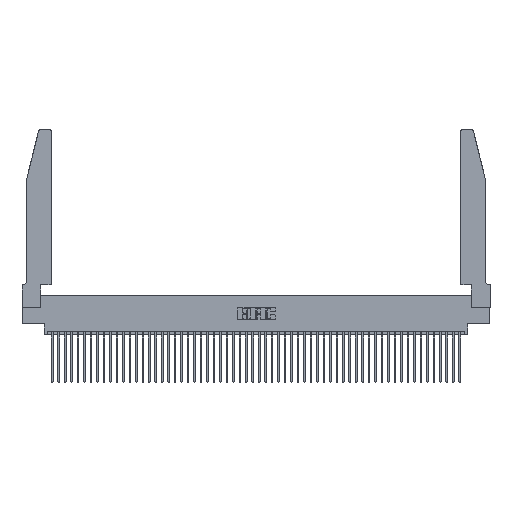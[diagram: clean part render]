
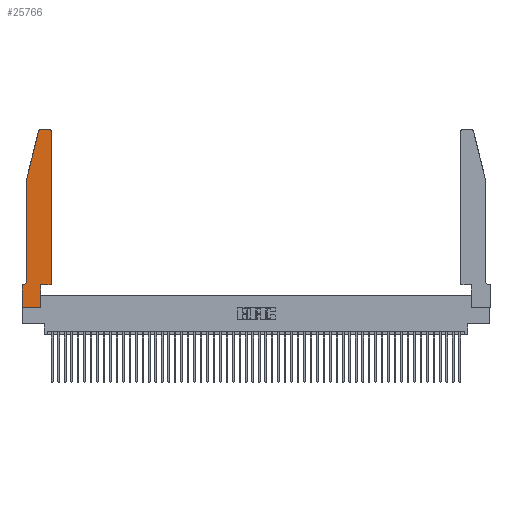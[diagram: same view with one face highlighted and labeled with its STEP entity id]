
A CAD part, top view. The second image highlights one B-rep face of the part: STEP entity #25766.
In plain terms, the highlighted planar face has unit normal (0, 0, 1).
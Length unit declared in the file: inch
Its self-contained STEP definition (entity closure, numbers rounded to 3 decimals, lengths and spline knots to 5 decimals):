
#330 = DIRECTION ( 'NONE',  ( 0., 0., 1. ) ) ;
#404 = VECTOR ( 'NONE', #18850, 39.37008 ) ;
#781 = CARTESIAN_POINT ( 'NONE',  ( 0.284, 2.75, 0.37 ) ) ;
#1384 = CIRCLE ( 'NONE', #18225, 0.03 ) ;
#3979 = EDGE_CURVE ( 'NONE', #7388, #43879, #4180, .T. ) ;
#4016 = VERTEX_POINT ( 'NONE', #40370 ) ;
#4180 = LINE ( 'NONE', #6668, #404 ) ;
#4726 = VECTOR ( 'NONE', #18629, 39.37008 ) ;
#5126 = DIRECTION ( 'NONE',  ( 1., 0., 0. ) ) ;
#5269 = EDGE_CURVE ( 'NONE', #43879, #4016, #16724, .T. ) ;
#5546 = CARTESIAN_POINT ( 'NONE',  ( 0., 0., 0.37 ) ) ;
#5637 = EDGE_CURVE ( 'NONE', #10008, #19108, #41903, .T. ) ;
#6426 = CARTESIAN_POINT ( 'NONE',  ( 0.0755, 2., 0.37 ) ) ;
#6668 = CARTESIAN_POINT ( 'NONE',  ( 0., 0., 0.37 ) ) ;
#7388 = VERTEX_POINT ( 'NONE', #5546 ) ;
#8539 = CARTESIAN_POINT ( 'NONE',  ( 0., 0., 0.37 ) ) ;
#9071 = VECTOR ( 'NONE', #16638, 39.37008 ) ;
#9257 = VERTEX_POINT ( 'NONE', #9500 ) ;
#9500 = CARTESIAN_POINT ( 'NONE',  ( 0.25487, 2.72718, 0.37 ) ) ;
#10008 = VERTEX_POINT ( 'NONE', #10995 ) ;
#10995 = CARTESIAN_POINT ( 'NONE',  ( 0.0755, 2., 0.37 ) ) ;
#12994 = CARTESIAN_POINT ( 'NONE',  ( 0.4505, 0.35, 0.37 ) ) ;
#13196 = EDGE_CURVE ( 'NONE', #45973, #7388, #28030, .T. ) ;
#13415 = LINE ( 'NONE', #6426, #45569 ) ;
#13963 = CARTESIAN_POINT ( 'NONE',  ( 0.4505, 0.35, 0.37 ) ) ;
#15102 = VERTEX_POINT ( 'NONE', #12994 ) ;
#15678 = LINE ( 'NONE', #13963, #29575 ) ;
#16039 = PLANE ( 'NONE',  #35941 ) ;
#16638 = DIRECTION ( 'NONE',  ( 0., -1., 0. ) ) ;
#16724 = LINE ( 'NONE', #31027, #38781 ) ;
#18225 = AXIS2_PLACEMENT_3D ( 'NONE', #20105, #48256, #39664 ) ;
#18579 = EDGE_CURVE ( 'NONE', #4016, #15102, #15678, .T. ) ;
#18629 = DIRECTION ( 'NONE',  ( 0., 1., 0. ) ) ;
#18850 = DIRECTION ( 'NONE',  ( 1., 0., 0. ) ) ;
#19108 = VERTEX_POINT ( 'NONE', #32781 ) ;
#19529 = ORIENTED_EDGE ( 'NONE', *, *, #46362, .T. ) ;
#20105 = CARTESIAN_POINT ( 'NONE',  ( 0.4205, 2.72, 0.37 ) ) ;
#20370 = EDGE_CURVE ( 'NONE', #15102, #50865, #33173, .T. ) ;
#21118 = DIRECTION ( 'NONE',  ( 0., 0., -1. ) ) ;
#21936 = CARTESIAN_POINT ( 'NONE',  ( 0.2865, 0., 0.37 ) ) ;
#22093 = CIRCLE ( 'NONE', #30400, 0.03 ) ;
#22524 = FACE_OUTER_BOUND ( 'NONE', #35643, .T. ) ;
#23201 = CARTESIAN_POINT ( 'NONE',  ( 0.4505, 0.35, 0.37 ) ) ;
#23268 = LINE ( 'NONE', #24668, #50334 ) ;
#23307 = ORIENTED_EDGE ( 'NONE', *, *, #3979, .T. ) ;
#23380 = ORIENTED_EDGE ( 'NONE', *, *, #32424, .T. ) ;
#24668 = CARTESIAN_POINT ( 'NONE',  ( 0.0755, 0.35, 0.37 ) ) ;
#24765 = DIRECTION ( 'NONE',  ( 1., 0., 0. ) ) ;
#24830 = CARTESIAN_POINT ( 'NONE',  ( 0.0055, 0.42, 0.37 ) ) ;
#25766 = ADVANCED_FACE ( 'NONE', ( #22524 ), #16039, .T. ) ;
#25947 = ORIENTED_EDGE ( 'NONE', *, *, #36126, .T. ) ;
#27326 = VERTEX_POINT ( 'NONE', #27696 ) ;
#27396 = VECTOR ( 'NONE', #48413, 39.37008 ) ;
#27696 = CARTESIAN_POINT ( 'NONE',  ( 0.0055, 0.35, 0.37 ) ) ;
#28030 = LINE ( 'NONE', #8539, #9071 ) ;
#29566 = ORIENTED_EDGE ( 'NONE', *, *, #5269, .T. ) ;
#29575 = VECTOR ( 'NONE', #5126, 39.37008 ) ;
#30163 = VERTEX_POINT ( 'NONE', #35203 ) ;
#30400 = AXIS2_PLACEMENT_3D ( 'NONE', #39882, #51823, #24765 ) ;
#30762 = DIRECTION ( 'NONE',  ( -0.239, -0.971, 0. ) ) ;
#31027 = CARTESIAN_POINT ( 'NONE',  ( 0.2865, 0.35, 0.37 ) ) ;
#31483 = EDGE_CURVE ( 'NONE', #50865, #30163, #1384, .T. ) ;
#31693 = ORIENTED_EDGE ( 'NONE', *, *, #13196, .T. ) ;
#32424 = EDGE_CURVE ( 'NONE', #52123, #9257, #22093, .T. ) ;
#32657 = CARTESIAN_POINT ( 'NONE',  ( 0.4505, 2.72, 0.37 ) ) ;
#32781 = CARTESIAN_POINT ( 'NONE',  ( 0.0755, 0.42, 0.37 ) ) ;
#32923 = DIRECTION ( 'NONE',  ( -1., 0., 0. ) ) ;
#33173 = LINE ( 'NONE', #23201, #4726 ) ;
#35203 = CARTESIAN_POINT ( 'NONE',  ( 0.4205, 2.75, 0.37 ) ) ;
#35643 = EDGE_LOOP ( 'NONE', ( #25947, #23380, #42198, #50506, #36216, #19529, #31693, #23307, #29566, #48095, #47998, #37978 ) ) ;
#35941 = AXIS2_PLACEMENT_3D ( 'NONE', #39837, #330, #40186 ) ;
#36126 = EDGE_CURVE ( 'NONE', #30163, #52123, #40978, .T. ) ;
#36216 = ORIENTED_EDGE ( 'NONE', *, *, #38710, .T. ) ;
#36310 = CARTESIAN_POINT ( 'NONE',  ( 0.0755, 2., 0.37 ) ) ;
#36649 = AXIS2_PLACEMENT_3D ( 'NONE', #24830, #21118, #32923 ) ;
#37978 = ORIENTED_EDGE ( 'NONE', *, *, #31483, .T. ) ;
#37987 = DIRECTION ( 'NONE',  ( -1., 0., 0. ) ) ;
#38158 = CARTESIAN_POINT ( 'NONE',  ( 0.2605, 2.75, 0.37 ) ) ;
#38710 = EDGE_CURVE ( 'NONE', #19108, #27326, #40685, .T. ) ;
#38781 = VECTOR ( 'NONE', #51425, 39.37008 ) ;
#39664 = DIRECTION ( 'NONE',  ( 1., 0., 0. ) ) ;
#39837 = CARTESIAN_POINT ( 'NONE',  ( 0., 0.35, 0.37 ) ) ;
#39882 = CARTESIAN_POINT ( 'NONE',  ( 0.284, 2.72, 0.37 ) ) ;
#40186 = DIRECTION ( 'NONE',  ( 1., 0., 0. ) ) ;
#40370 = CARTESIAN_POINT ( 'NONE',  ( 0.2865, 0.35, 0.37 ) ) ;
#40685 = CIRCLE ( 'NONE', #36649, 0.07 ) ;
#40978 = LINE ( 'NONE', #38158, #45390 ) ;
#41903 = LINE ( 'NONE', #36310, #27396 ) ;
#42198 = ORIENTED_EDGE ( 'NONE', *, *, #50404, .T. ) ;
#43879 = VERTEX_POINT ( 'NONE', #21936 ) ;
#44535 = DIRECTION ( 'NONE',  ( -1., 0., 0. ) ) ;
#45390 = VECTOR ( 'NONE', #37987, 39.37008 ) ;
#45569 = VECTOR ( 'NONE', #30762, 39.37008 ) ;
#45973 = VERTEX_POINT ( 'NONE', #50737 ) ;
#46362 = EDGE_CURVE ( 'NONE', #27326, #45973, #23268, .T. ) ;
#47998 = ORIENTED_EDGE ( 'NONE', *, *, #20370, .T. ) ;
#48095 = ORIENTED_EDGE ( 'NONE', *, *, #18579, .T. ) ;
#48256 = DIRECTION ( 'NONE',  ( 0., 0., 1. ) ) ;
#48413 = DIRECTION ( 'NONE',  ( 0., -1., 0. ) ) ;
#50334 = VECTOR ( 'NONE', #44535, 39.37008 ) ;
#50404 = EDGE_CURVE ( 'NONE', #9257, #10008, #13415, .T. ) ;
#50506 = ORIENTED_EDGE ( 'NONE', *, *, #5637, .T. ) ;
#50737 = CARTESIAN_POINT ( 'NONE',  ( 0., 0.35, 0.37 ) ) ;
#50865 = VERTEX_POINT ( 'NONE', #32657 ) ;
#51425 = DIRECTION ( 'NONE',  ( 0., 1., 0. ) ) ;
#51823 = DIRECTION ( 'NONE',  ( 0., 0., 1. ) ) ;
#52123 = VERTEX_POINT ( 'NONE', #781 ) ;
